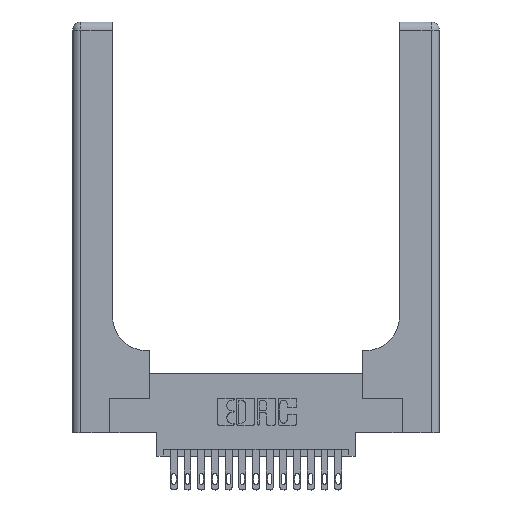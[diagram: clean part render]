
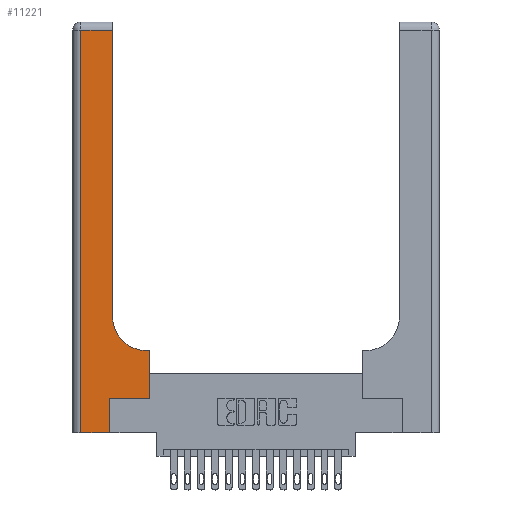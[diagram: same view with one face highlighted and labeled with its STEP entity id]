
A CAD part, top view. The second image highlights one B-rep face of the part: STEP entity #11221.
In plain terms, the highlighted planar face has unit normal (0, 0, 1).
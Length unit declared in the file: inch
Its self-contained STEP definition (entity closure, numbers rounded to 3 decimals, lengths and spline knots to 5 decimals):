
#342 = LINE ( 'NONE', #9119, #13902 ) ;
#496 = AXIS2_PLACEMENT_3D ( 'NONE', #1139, #4335, #16100 ) ;
#1139 = CARTESIAN_POINT ( 'NONE',  ( 0.5415, 0.85, 0.37 ) ) ;
#1553 = EDGE_CURVE ( 'NONE', #16259, #11123, #7512, .T. ) ;
#1586 = VERTEX_POINT ( 'NONE', #2047 ) ;
#1811 = DIRECTION ( 'NONE',  ( 0., 1., 0. ) ) ;
#2047 = CARTESIAN_POINT ( 'NONE',  ( 0.2915, 0.85, 0.37 ) ) ;
#2055 = CARTESIAN_POINT ( 'NONE',  ( 0.269, 0.25, 0.37 ) ) ;
#2473 = DIRECTION ( 'NONE',  ( -1., 0., 0. ) ) ;
#3857 = ORIENTED_EDGE ( 'NONE', *, *, #7986, .T. ) ;
#4335 = DIRECTION ( 'NONE',  ( 0., 0., -1. ) ) ;
#4854 = ORIENTED_EDGE ( 'NONE', *, *, #17228, .T. ) ;
#4976 = VERTEX_POINT ( 'NONE', #2055 ) ;
#5040 = CARTESIAN_POINT ( 'NONE',  ( 0.2915, 2.94, 0.37 ) ) ;
#5570 = DIRECTION ( 'NONE',  ( 1., 0., 0. ) ) ;
#5640 = VECTOR ( 'NONE', #5570, 39.37008 ) ;
#6190 = ORIENTED_EDGE ( 'NONE', *, *, #13012, .T. ) ;
#6447 = DIRECTION ( 'NONE',  ( 0., 1., 0. ) ) ;
#6698 = CARTESIAN_POINT ( 'NONE',  ( 0.2915, 0.6, 0.37 ) ) ;
#7298 = ORIENTED_EDGE ( 'NONE', *, *, #1553, .T. ) ;
#7346 = CARTESIAN_POINT ( 'NONE',  ( 0., 0., 0.37 ) ) ;
#7425 = DIRECTION ( 'NONE',  ( 0., 1., 0. ) ) ;
#7512 = LINE ( 'NONE', #15361, #10092 ) ;
#7666 = FACE_OUTER_BOUND ( 'NONE', #12789, .T. ) ;
#7986 = EDGE_CURVE ( 'NONE', #12513, #14003, #14589, .T. ) ;
#8214 = ORIENTED_EDGE ( 'NONE', *, *, #18492, .T. ) ;
#8305 = VERTEX_POINT ( 'NONE', #12065 ) ;
#8854 = ORIENTED_EDGE ( 'NONE', *, *, #17286, .T. ) ;
#9119 = CARTESIAN_POINT ( 'NONE',  ( 0.06, 3., 0.37 ) ) ;
#9207 = AXIS2_PLACEMENT_3D ( 'NONE', #16831, #16765, #15350 ) ;
#9219 = CARTESIAN_POINT ( 'NONE',  ( 0.5585, 0.25, 0.37 ) ) ;
#9423 = ORIENTED_EDGE ( 'NONE', *, *, #19127, .T. ) ;
#9490 = CARTESIAN_POINT ( 'NONE',  ( 0.5585, 0.6, 0.37 ) ) ;
#9663 = LINE ( 'NONE', #7346, #14801 ) ;
#10092 = VECTOR ( 'NONE', #16910, 39.37008 ) ;
#10528 = CARTESIAN_POINT ( 'NONE',  ( 0.06, 2.94, 0.37 ) ) ;
#10664 = LINE ( 'NONE', #9219, #18142 ) ;
#11123 = VERTEX_POINT ( 'NONE', #10528 ) ;
#11221 = ADVANCED_FACE ( 'NONE', ( #7666 ), #13595, .F. ) ;
#11427 = DIRECTION ( 'NONE',  ( 0., -1., 0. ) ) ;
#11970 = LINE ( 'NONE', #12375, #15461 ) ;
#12065 = CARTESIAN_POINT ( 'NONE',  ( 0.5585, 0.25, 0.37 ) ) ;
#12375 = CARTESIAN_POINT ( 'NONE',  ( 0.269, 0., 0.37 ) ) ;
#12513 = VERTEX_POINT ( 'NONE', #9490 ) ;
#12789 = EDGE_LOOP ( 'NONE', ( #8214, #7298, #18524, #8854, #9423, #14858, #6190, #3857, #4854 ) ) ;
#13012 = EDGE_CURVE ( 'NONE', #8305, #12513, #10664, .T. ) ;
#13141 = VECTOR ( 'NONE', #7425, 39.37008 ) ;
#13240 = VERTEX_POINT ( 'NONE', #17367 ) ;
#13408 = VECTOR ( 'NONE', #2473, 39.37008 ) ;
#13595 = PLANE ( 'NONE',  #9207 ) ;
#13651 = CARTESIAN_POINT ( 'NONE',  ( 0.269, 0., 0.37 ) ) ;
#13902 = VECTOR ( 'NONE', #11427, 39.37008 ) ;
#14003 = VERTEX_POINT ( 'NONE', #16819 ) ;
#14564 = LINE ( 'NONE', #16306, #13141 ) ;
#14589 = LINE ( 'NONE', #6698, #13408 ) ;
#14801 = VECTOR ( 'NONE', #17793, 39.37008 ) ;
#14858 = ORIENTED_EDGE ( 'NONE', *, *, #19046, .T. ) ;
#15032 = CIRCLE ( 'NONE', #496, 0.25 ) ;
#15350 = DIRECTION ( 'NONE',  ( -1., 0., 0. ) ) ;
#15361 = CARTESIAN_POINT ( 'NONE',  ( 0., 2.94, 0.37 ) ) ;
#15461 = VECTOR ( 'NONE', #1811, 39.37008 ) ;
#16011 = EDGE_CURVE ( 'NONE', #11123, #13240, #342, .T. ) ;
#16100 = DIRECTION ( 'NONE',  ( 1., 0., 0. ) ) ;
#16259 = VERTEX_POINT ( 'NONE', #5040 ) ;
#16306 = CARTESIAN_POINT ( 'NONE',  ( 0.2915, 3., 0.37 ) ) ;
#16765 = DIRECTION ( 'NONE',  ( 0., 0., -1. ) ) ;
#16819 = CARTESIAN_POINT ( 'NONE',  ( 0.5415, 0.6, 0.37 ) ) ;
#16831 = CARTESIAN_POINT ( 'NONE',  ( 0., 3., 0.37 ) ) ;
#16910 = DIRECTION ( 'NONE',  ( -1., 0., 0. ) ) ;
#17228 = EDGE_CURVE ( 'NONE', #14003, #1586, #15032, .T. ) ;
#17286 = EDGE_CURVE ( 'NONE', #13240, #17947, #9663, .T. ) ;
#17367 = CARTESIAN_POINT ( 'NONE',  ( 0.06, 0., 0.37 ) ) ;
#17718 = CARTESIAN_POINT ( 'NONE',  ( 0.269, 0.25, 0.37 ) ) ;
#17793 = DIRECTION ( 'NONE',  ( 1., 0., 0. ) ) ;
#17947 = VERTEX_POINT ( 'NONE', #13651 ) ;
#18142 = VECTOR ( 'NONE', #6447, 39.37008 ) ;
#18492 = EDGE_CURVE ( 'NONE', #1586, #16259, #14564, .T. ) ;
#18500 = LINE ( 'NONE', #17718, #5640 ) ;
#18524 = ORIENTED_EDGE ( 'NONE', *, *, #16011, .T. ) ;
#19046 = EDGE_CURVE ( 'NONE', #4976, #8305, #18500, .T. ) ;
#19127 = EDGE_CURVE ( 'NONE', #17947, #4976, #11970, .T. ) ;
